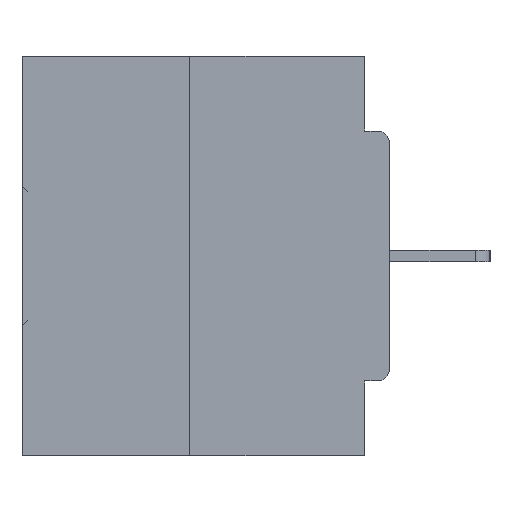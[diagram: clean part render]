
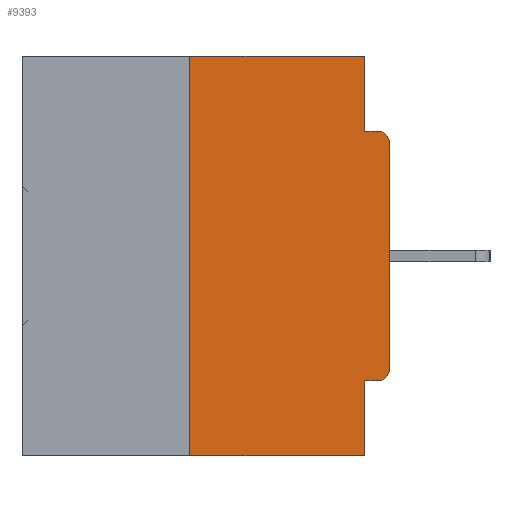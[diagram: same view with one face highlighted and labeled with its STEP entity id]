
A CAD part, left-side view. The second image highlights one B-rep face of the part: STEP entity #9393.
In plain terms, the highlighted planar face has unit normal (-1, 0, 0).
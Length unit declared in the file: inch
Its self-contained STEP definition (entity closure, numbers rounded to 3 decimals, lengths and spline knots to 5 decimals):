
#1076 = CARTESIAN_POINT ( 'NONE',  ( 0., 0.031, 0. ) ) ;
#1277 = DIRECTION ( 'NONE',  ( 0., 0., -1. ) ) ;
#1368 = CARTESIAN_POINT ( 'NONE',  ( 0., 0.015, -0.3915 ) ) ;
#1798 = DIRECTION ( 'NONE',  ( -1., 0., 0. ) ) ;
#3062 = DIRECTION ( 'NONE',  ( 0., 0., -1. ) ) ;
#4088 = DIRECTION ( 'NONE',  ( 1., 0., 0. ) ) ;
#4825 = CARTESIAN_POINT ( 'NONE',  ( 0., 0.46, -0.5 ) ) ;
#4859 = LINE ( 'NONE', #25863, #25614 ) ;
#5068 = CIRCLE ( 'NONE', #27907, 0.015 ) ;
#5342 = CARTESIAN_POINT ( 'NONE',  ( 0., 0.031, -0.5 ) ) ;
#5873 = EDGE_CURVE ( 'NONE', #27550, #27450, #12239, .T. ) ;
#6246 = DIRECTION ( 'NONE',  ( -1., 0., 0. ) ) ;
#6533 = VERTEX_POINT ( 'NONE', #5342 ) ;
#6911 = AXIS2_PLACEMENT_3D ( 'NONE', #1368, #1798, #8063 ) ;
#7630 = EDGE_CURVE ( 'NONE', #27450, #6533, #20279, .T. ) ;
#8063 = DIRECTION ( 'NONE',  ( 0., 0., -1. ) ) ;
#9190 = AXIS2_PLACEMENT_3D ( 'NONE', #19837, #4088, #1277 ) ;
#9393 = ADVANCED_FACE ( 'NONE', ( #31570 ), #13647, .F. ) ;
#9664 = LINE ( 'NONE', #4825, #38396 ) ;
#12239 = LINE ( 'NONE', #30216, #20644 ) ;
#12362 = VECTOR ( 'NONE', #21545, 39.37008 ) ;
#13425 = CARTESIAN_POINT ( 'NONE',  ( 0., 0.015, -0.0935 ) ) ;
#13647 = PLANE ( 'NONE',  #9190 ) ;
#13694 = CARTESIAN_POINT ( 'NONE',  ( 0., 0., -0.0935 ) ) ;
#13851 = VERTEX_POINT ( 'NONE', #18799 ) ;
#14210 = VERTEX_POINT ( 'NONE', #21695 ) ;
#14320 = VECTOR ( 'NONE', #22146, 39.37008 ) ;
#15968 = CARTESIAN_POINT ( 'NONE',  ( 0., 0.015, -0.4065 ) ) ;
#16712 = CARTESIAN_POINT ( 'NONE',  ( 0., 0.25, -0.5 ) ) ;
#18183 = ORIENTED_EDGE ( 'NONE', *, *, #39067, .F. ) ;
#18397 = EDGE_CURVE ( 'NONE', #34441, #6533, #9664, .T. ) ;
#18799 = CARTESIAN_POINT ( 'NONE',  ( 0., 0.25, 0. ) ) ;
#18849 = EDGE_CURVE ( 'NONE', #27550, #21845, #29446, .T. ) ;
#19837 = CARTESIAN_POINT ( 'NONE',  ( 0., 0.46, 0. ) ) ;
#20001 = EDGE_CURVE ( 'NONE', #14210, #25062, #5068, .T. ) ;
#20279 = LINE ( 'NONE', #27660, #12362 ) ;
#20644 = VECTOR ( 'NONE', #36731, 39.37008 ) ;
#20910 = DIRECTION ( 'NONE',  ( 0., 0., 1. ) ) ;
#21066 = EDGE_CURVE ( 'NONE', #21845, #14210, #36183, .T. ) ;
#21545 = DIRECTION ( 'NONE',  ( 0., 0., -1. ) ) ;
#21695 = CARTESIAN_POINT ( 'NONE',  ( 0., 0., -0.1085 ) ) ;
#21845 = VERTEX_POINT ( 'NONE', #35971 ) ;
#22146 = DIRECTION ( 'NONE',  ( 0., 0., -1. ) ) ;
#23414 = ORIENTED_EDGE ( 'NONE', *, *, #30984, .F. ) ;
#24931 = CARTESIAN_POINT ( 'NONE',  ( 0., 0.031, 0. ) ) ;
#24960 = LINE ( 'NONE', #30319, #40857 ) ;
#25062 = VERTEX_POINT ( 'NONE', #13425 ) ;
#25614 = VECTOR ( 'NONE', #25729, 39.37008 ) ;
#25688 = LINE ( 'NONE', #24931, #14320 ) ;
#25729 = DIRECTION ( 'NONE',  ( 0., -1., 0. ) ) ;
#25863 = CARTESIAN_POINT ( 'NONE',  ( 0., 0.46, 0. ) ) ;
#26237 = ORIENTED_EDGE ( 'NONE', *, *, #31671, .F. ) ;
#27450 = VERTEX_POINT ( 'NONE', #37605 ) ;
#27550 = VERTEX_POINT ( 'NONE', #15968 ) ;
#27660 = CARTESIAN_POINT ( 'NONE',  ( 0., 0.031, -0.5 ) ) ;
#27775 = ORIENTED_EDGE ( 'NONE', *, *, #20001, .T. ) ;
#27825 = CARTESIAN_POINT ( 'NONE',  ( 0., 0., 0. ) ) ;
#27907 = AXIS2_PLACEMENT_3D ( 'NONE', #32020, #6246, #3062 ) ;
#28357 = CARTESIAN_POINT ( 'NONE',  ( 0., 0.031, -0.0935 ) ) ;
#29256 = VECTOR ( 'NONE', #20910, 39.37008 ) ;
#29446 = CIRCLE ( 'NONE', #6911, 0.015 ) ;
#29946 = VERTEX_POINT ( 'NONE', #1076 ) ;
#30035 = ORIENTED_EDGE ( 'NONE', *, *, #21066, .T. ) ;
#30046 = DIRECTION ( 'NONE',  ( 0., 0., 1. ) ) ;
#30216 = CARTESIAN_POINT ( 'NONE',  ( 0., 0., -0.4065 ) ) ;
#30319 = CARTESIAN_POINT ( 'NONE',  ( 0., 0.25, 0. ) ) ;
#30984 = EDGE_CURVE ( 'NONE', #29946, #32530, #25688, .T. ) ;
#31570 = FACE_OUTER_BOUND ( 'NONE', #38793, .T. ) ;
#31671 = EDGE_CURVE ( 'NONE', #13851, #29946, #4859, .T. ) ;
#32020 = CARTESIAN_POINT ( 'NONE',  ( 0., 0.015, -0.1085 ) ) ;
#32472 = LINE ( 'NONE', #13694, #40929 ) ;
#32530 = VERTEX_POINT ( 'NONE', #28357 ) ;
#33757 = ORIENTED_EDGE ( 'NONE', *, *, #18849, .T. ) ;
#34399 = ORIENTED_EDGE ( 'NONE', *, *, #37450, .F. ) ;
#34441 = VERTEX_POINT ( 'NONE', #16712 ) ;
#34837 = ORIENTED_EDGE ( 'NONE', *, *, #5873, .F. ) ;
#35835 = DIRECTION ( 'NONE',  ( 0., -1., 0. ) ) ;
#35963 = ORIENTED_EDGE ( 'NONE', *, *, #18397, .T. ) ;
#35971 = CARTESIAN_POINT ( 'NONE',  ( 0., 0., -0.3915 ) ) ;
#36183 = LINE ( 'NONE', #27825, #29256 ) ;
#36393 = DIRECTION ( 'NONE',  ( 0., -1., 0. ) ) ;
#36731 = DIRECTION ( 'NONE',  ( 0., 1., 0. ) ) ;
#37450 = EDGE_CURVE ( 'NONE', #32530, #25062, #32472, .T. ) ;
#37605 = CARTESIAN_POINT ( 'NONE',  ( 0., 0.031, -0.4065 ) ) ;
#38396 = VECTOR ( 'NONE', #36393, 39.37008 ) ;
#38793 = EDGE_LOOP ( 'NONE', ( #26237, #18183, #35963, #41059, #34837, #33757, #30035, #27775, #34399, #23414 ) ) ;
#39067 = EDGE_CURVE ( 'NONE', #34441, #13851, #24960, .T. ) ;
#40857 = VECTOR ( 'NONE', #30046, 39.37008 ) ;
#40929 = VECTOR ( 'NONE', #35835, 39.37008 ) ;
#41059 = ORIENTED_EDGE ( 'NONE', *, *, #7630, .F. ) ;
